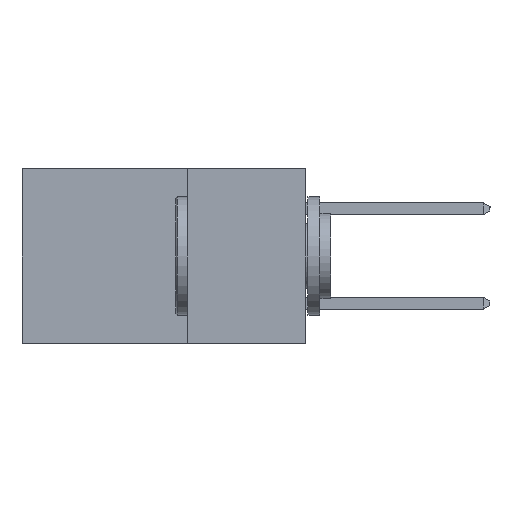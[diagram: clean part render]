
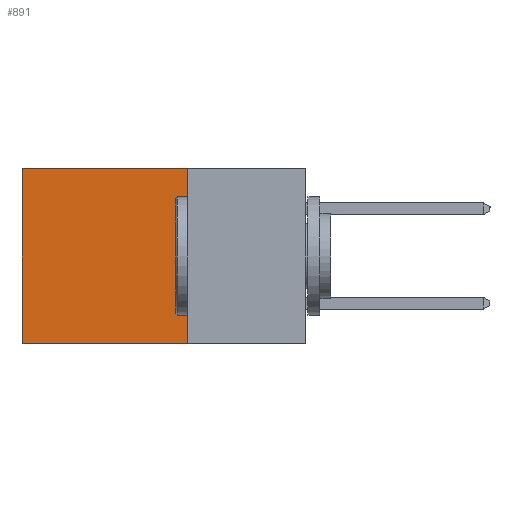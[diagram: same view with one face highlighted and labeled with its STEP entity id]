
A CAD part, left-side view. The second image highlights one B-rep face of the part: STEP entity #891.
In plain terms, the highlighted planar face has unit normal (-1, 0, 0).
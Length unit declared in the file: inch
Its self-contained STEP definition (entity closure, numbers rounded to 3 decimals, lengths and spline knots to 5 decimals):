
#76 = CARTESIAN_POINT ( 'NONE',  ( 0.2615, 0.25, -0.37 ) ) ;
#525 = EDGE_CURVE ( 'NONE', #1971, #7240, #11090, .T. ) ;
#580 = VECTOR ( 'NONE', #4017, 39.37008 ) ;
#682 = LINE ( 'NONE', #2717, #3902 ) ;
#795 = DIRECTION ( 'NONE',  ( 1., 0., 0. ) ) ;
#871 = LINE ( 'NONE', #8946, #580 ) ;
#891 = ADVANCED_FACE ( 'NONE', ( #8534 ), #3430, .F. ) ;
#1288 = CARTESIAN_POINT ( 'NONE',  ( 0.2615, 0.6, 0. ) ) ;
#1522 = VECTOR ( 'NONE', #3366, 39.37008 ) ;
#1971 = VERTEX_POINT ( 'NONE', #1288 ) ;
#2233 = VERTEX_POINT ( 'NONE', #2900 ) ;
#2443 = LINE ( 'NONE', #5502, #1522 ) ;
#2716 = ORIENTED_EDGE ( 'NONE', *, *, #3391, .T. ) ;
#2717 = CARTESIAN_POINT ( 'NONE',  ( 0.2615, 0.25, -0.37 ) ) ;
#2900 = CARTESIAN_POINT ( 'NONE',  ( 0.2615, 0.25, 0. ) ) ;
#3366 = DIRECTION ( 'NONE',  ( 0., 1., 0. ) ) ;
#3391 = EDGE_CURVE ( 'NONE', #2233, #1971, #2443, .T. ) ;
#3430 = PLANE ( 'NONE',  #6219 ) ;
#3579 = EDGE_CURVE ( 'NONE', #4107, #7240, #682, .T. ) ;
#3629 = ORIENTED_EDGE ( 'NONE', *, *, #3579, .F. ) ;
#3902 = VECTOR ( 'NONE', #6591, 39.37008 ) ;
#4017 = DIRECTION ( 'NONE',  ( 0., 0., -1. ) ) ;
#4107 = VERTEX_POINT ( 'NONE', #76 ) ;
#4964 = VECTOR ( 'NONE', #11211, 39.37008 ) ;
#5502 = CARTESIAN_POINT ( 'NONE',  ( 0.2615, 0.25, 0. ) ) ;
#6111 = EDGE_CURVE ( 'NONE', #2233, #4107, #871, .T. ) ;
#6219 = AXIS2_PLACEMENT_3D ( 'NONE', #7525, #795, #6962 ) ;
#6591 = DIRECTION ( 'NONE',  ( 0., 1., 0. ) ) ;
#6823 = CARTESIAN_POINT ( 'NONE',  ( 0.2615, 0.6, -0.37 ) ) ;
#6962 = DIRECTION ( 'NONE',  ( 0., 0., -1. ) ) ;
#7240 = VERTEX_POINT ( 'NONE', #6823 ) ;
#7525 = CARTESIAN_POINT ( 'NONE',  ( 0.2615, 0.25, -0.37 ) ) ;
#8534 = FACE_OUTER_BOUND ( 'NONE', #11497, .T. ) ;
#8946 = CARTESIAN_POINT ( 'NONE',  ( 0.2615, 0.25, -0.37 ) ) ;
#10414 = ORIENTED_EDGE ( 'NONE', *, *, #525, .T. ) ;
#10555 = ORIENTED_EDGE ( 'NONE', *, *, #6111, .F. ) ;
#11090 = LINE ( 'NONE', #12160, #4964 ) ;
#11211 = DIRECTION ( 'NONE',  ( 0., 0., -1. ) ) ;
#11497 = EDGE_LOOP ( 'NONE', ( #10414, #3629, #10555, #2716 ) ) ;
#12160 = CARTESIAN_POINT ( 'NONE',  ( 0.2615, 0.6, -0.37 ) ) ;
